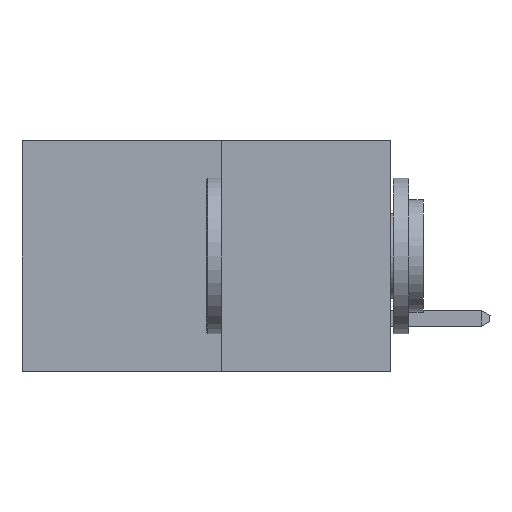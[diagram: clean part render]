
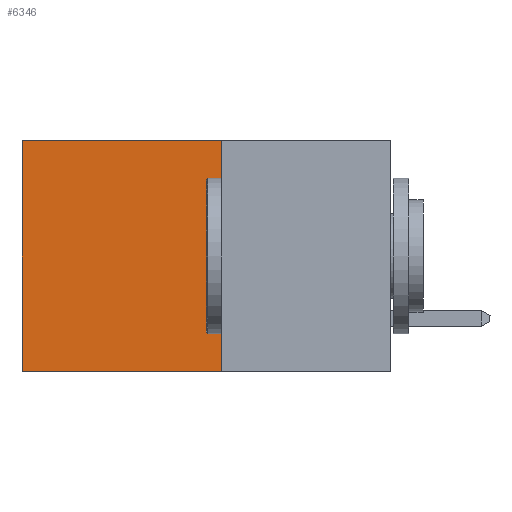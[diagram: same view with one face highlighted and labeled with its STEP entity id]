
A CAD part, left-side view. The second image highlights one B-rep face of the part: STEP entity #6346.
In plain terms, the highlighted planar face has unit normal (-1, 0, 0).
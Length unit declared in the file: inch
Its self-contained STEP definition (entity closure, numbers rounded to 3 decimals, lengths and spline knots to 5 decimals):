
#43 = EDGE_CURVE ( 'NONE', #5429, #5240, #2964, .T. ) ;
#156 = LINE ( 'NONE', #4980, #4543 ) ;
#332 = VECTOR ( 'NONE', #10144, 39.37008 ) ;
#607 = DIRECTION ( 'NONE',  ( 0., 0., -1. ) ) ;
#613 = DIRECTION ( 'NONE',  ( 1., 0., 0. ) ) ;
#626 = DIRECTION ( 'NONE',  ( 0., 0., -1. ) ) ;
#654 = EDGE_CURVE ( 'NONE', #5124, #6523, #3928, .T. ) ;
#670 = CARTESIAN_POINT ( 'NONE',  ( 0.277, 0.27, -0.37 ) ) ;
#1020 = PLANE ( 'NONE',  #4982 ) ;
#2787 = CARTESIAN_POINT ( 'NONE',  ( 0.277, 0.27, 0. ) ) ;
#2925 = ORIENTED_EDGE ( 'NONE', *, *, #6895, .T. ) ;
#2964 = LINE ( 'NONE', #3421, #5026 ) ;
#3282 = FACE_OUTER_BOUND ( 'NONE', #6477, .T. ) ;
#3421 = CARTESIAN_POINT ( 'NONE',  ( 0.277, 0.27, -0.37 ) ) ;
#3454 = CARTESIAN_POINT ( 'NONE',  ( 0.277, 0.59, 0. ) ) ;
#3521 = EDGE_CURVE ( 'NONE', #5240, #6523, #7134, .T. ) ;
#3864 = CARTESIAN_POINT ( 'NONE',  ( 0.277, 0.27, -0.37 ) ) ;
#3928 = LINE ( 'NONE', #8936, #5886 ) ;
#4543 = VECTOR ( 'NONE', #4940, 39.37008 ) ;
#4940 = DIRECTION ( 'NONE',  ( 0., 1., 0. ) ) ;
#4980 = CARTESIAN_POINT ( 'NONE',  ( 0.277, 0.27, 0. ) ) ;
#4982 = AXIS2_PLACEMENT_3D ( 'NONE', #670, #613, #626 ) ;
#5026 = VECTOR ( 'NONE', #5792, 39.37008 ) ;
#5124 = VERTEX_POINT ( 'NONE', #3454 ) ;
#5240 = VERTEX_POINT ( 'NONE', #3864 ) ;
#5429 = VERTEX_POINT ( 'NONE', #2787 ) ;
#5643 = ORIENTED_EDGE ( 'NONE', *, *, #3521, .F. ) ;
#5792 = DIRECTION ( 'NONE',  ( 0., 0., -1. ) ) ;
#5886 = VECTOR ( 'NONE', #607, 39.37008 ) ;
#6346 = ADVANCED_FACE ( 'NONE', ( #3282 ), #1020, .F. ) ;
#6477 = EDGE_LOOP ( 'NONE', ( #9190, #5643, #8484, #2925 ) ) ;
#6523 = VERTEX_POINT ( 'NONE', #9171 ) ;
#6895 = EDGE_CURVE ( 'NONE', #5429, #5124, #156, .T. ) ;
#7134 = LINE ( 'NONE', #10321, #332 ) ;
#8484 = ORIENTED_EDGE ( 'NONE', *, *, #43, .F. ) ;
#8936 = CARTESIAN_POINT ( 'NONE',  ( 0.277, 0.59, -0.37 ) ) ;
#9171 = CARTESIAN_POINT ( 'NONE',  ( 0.277, 0.59, -0.37 ) ) ;
#9190 = ORIENTED_EDGE ( 'NONE', *, *, #654, .T. ) ;
#10144 = DIRECTION ( 'NONE',  ( 0., 1., 0. ) ) ;
#10321 = CARTESIAN_POINT ( 'NONE',  ( 0.277, 0.27, -0.37 ) ) ;
